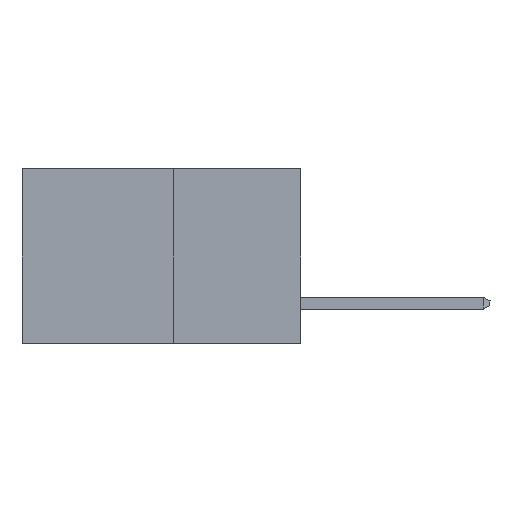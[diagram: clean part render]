
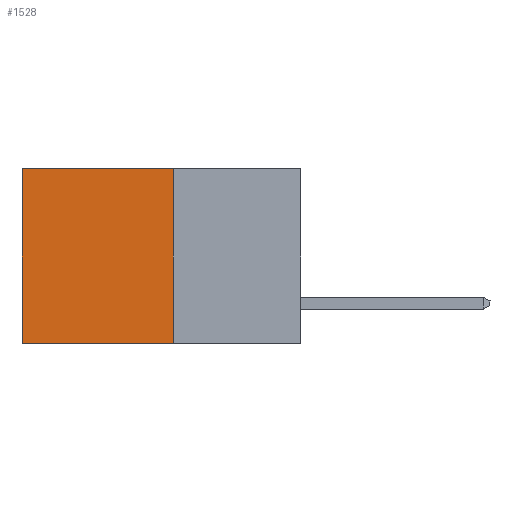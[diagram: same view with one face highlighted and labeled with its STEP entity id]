
A CAD part, left-side view. The second image highlights one B-rep face of the part: STEP entity #1528.
In plain terms, the highlighted planar face has unit normal (-1, 0, 0).
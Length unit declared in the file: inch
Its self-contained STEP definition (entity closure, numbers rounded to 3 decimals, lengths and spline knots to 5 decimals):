
#522 = LINE ( 'NONE', #6961, #6765 ) ;
#975 = CARTESIAN_POINT ( 'NONE',  ( 0.277, 0.27, -0.37 ) ) ;
#1085 = ORIENTED_EDGE ( 'NONE', *, *, #5046, .F. ) ;
#1162 = VERTEX_POINT ( 'NONE', #1613 ) ;
#1343 = DIRECTION ( 'NONE',  ( 0., 0., -1. ) ) ;
#1519 = LINE ( 'NONE', #8556, #10149 ) ;
#1528 = ADVANCED_FACE ( 'NONE', ( #5547 ), #2478, .F. ) ;
#1613 = CARTESIAN_POINT ( 'NONE',  ( 0.277, 0.27, 0. ) ) ;
#2478 = PLANE ( 'NONE',  #5296 ) ;
#2790 = DIRECTION ( 'NONE',  ( 0., 0., -1. ) ) ;
#2892 = EDGE_CURVE ( 'NONE', #9963, #6523, #522, .T. ) ;
#3027 = EDGE_CURVE ( 'NONE', #1162, #13877, #1519, .T. ) ;
#3541 = LINE ( 'NONE', #7608, #14333 ) ;
#3560 = LINE ( 'NONE', #10088, #10050 ) ;
#4868 = EDGE_CURVE ( 'NONE', #13877, #6523, #3541, .T. ) ;
#5046 = EDGE_CURVE ( 'NONE', #1162, #9963, #3560, .T. ) ;
#5171 = DIRECTION ( 'NONE',  ( 0., 1., 0. ) ) ;
#5296 = AXIS2_PLACEMENT_3D ( 'NONE', #975, #7949, #1343 ) ;
#5547 = FACE_OUTER_BOUND ( 'NONE', #7480, .T. ) ;
#5788 = CARTESIAN_POINT ( 'NONE',  ( 0.277, 0.27, -0.37 ) ) ;
#6523 = VERTEX_POINT ( 'NONE', #12279 ) ;
#6765 = VECTOR ( 'NONE', #5171, 39.37008 ) ;
#6961 = CARTESIAN_POINT ( 'NONE',  ( 0.277, 0.27, -0.37 ) ) ;
#7480 = EDGE_LOOP ( 'NONE', ( #11639, #12492, #1085, #9318 ) ) ;
#7608 = CARTESIAN_POINT ( 'NONE',  ( 0.277, 0.59, -0.37 ) ) ;
#7949 = DIRECTION ( 'NONE',  ( 1., 0., 0. ) ) ;
#8319 = CARTESIAN_POINT ( 'NONE',  ( 0.277, 0.59, 0. ) ) ;
#8556 = CARTESIAN_POINT ( 'NONE',  ( 0.277, 0.27, 0. ) ) ;
#9318 = ORIENTED_EDGE ( 'NONE', *, *, #3027, .T. ) ;
#9963 = VERTEX_POINT ( 'NONE', #5788 ) ;
#10050 = VECTOR ( 'NONE', #2790, 39.37008 ) ;
#10088 = CARTESIAN_POINT ( 'NONE',  ( 0.277, 0.27, -0.37 ) ) ;
#10149 = VECTOR ( 'NONE', #12552, 39.37008 ) ;
#11639 = ORIENTED_EDGE ( 'NONE', *, *, #4868, .T. ) ;
#12279 = CARTESIAN_POINT ( 'NONE',  ( 0.277, 0.59, -0.37 ) ) ;
#12324 = DIRECTION ( 'NONE',  ( 0., 0., -1. ) ) ;
#12492 = ORIENTED_EDGE ( 'NONE', *, *, #2892, .F. ) ;
#12552 = DIRECTION ( 'NONE',  ( 0., 1., 0. ) ) ;
#13877 = VERTEX_POINT ( 'NONE', #8319 ) ;
#14333 = VECTOR ( 'NONE', #12324, 39.37008 ) ;
